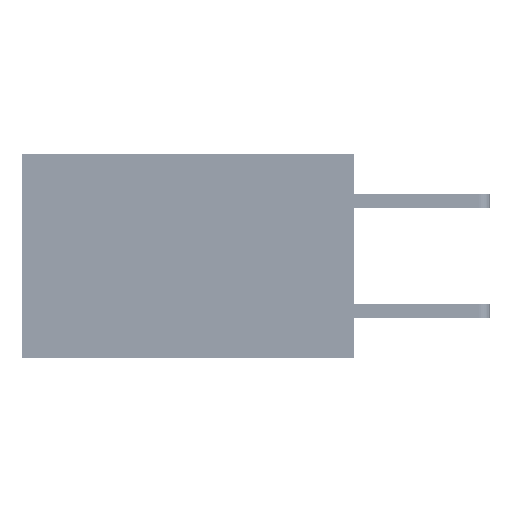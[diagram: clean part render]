
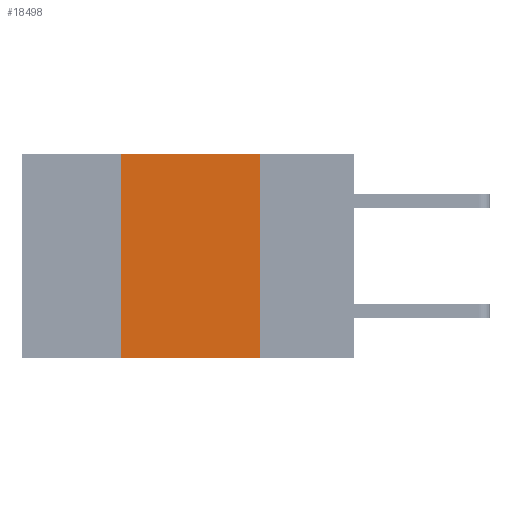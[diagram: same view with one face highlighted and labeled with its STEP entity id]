
A CAD part, left-side view. The second image highlights one B-rep face of the part: STEP entity #18498.
In plain terms, the highlighted planar face has unit normal (-1, 0, 0).
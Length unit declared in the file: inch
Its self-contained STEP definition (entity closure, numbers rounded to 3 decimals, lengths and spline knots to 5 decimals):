
#90 = LINE ( 'NONE', #34822, #17139 ) ;
#1323 = CARTESIAN_POINT ( 'NONE',  ( 0., 0.17, 0. ) ) ;
#3475 = DIRECTION ( 'NONE',  ( 1., 0., 0. ) ) ;
#3822 = EDGE_CURVE ( 'NONE', #50063, #41217, #90, .T. ) ;
#6707 = DIRECTION ( 'NONE',  ( 0., -1., 0. ) ) ;
#9091 = AXIS2_PLACEMENT_3D ( 'NONE', #14913, #3475, #50179 ) ;
#12660 = EDGE_CURVE ( 'NONE', #41217, #47361, #46963, .T. ) ;
#13399 = EDGE_CURVE ( 'NONE', #50063, #32348, #36809, .T. ) ;
#14913 = CARTESIAN_POINT ( 'NONE',  ( 0., 0.6, 0. ) ) ;
#15316 = DIRECTION ( 'NONE',  ( 0., -1., 0. ) ) ;
#17139 = VECTOR ( 'NONE', #49653, 39.37008 ) ;
#18024 = ORIENTED_EDGE ( 'NONE', *, *, #44090, .F. ) ;
#18498 = ADVANCED_FACE ( 'NONE', ( #37537 ), #22883, .F. ) ;
#22883 = PLANE ( 'NONE',  #9091 ) ;
#25505 = VECTOR ( 'NONE', #28757, 39.37008 ) ;
#26933 = CARTESIAN_POINT ( 'NONE',  ( 0., 0.42, -0.37 ) ) ;
#27983 = EDGE_LOOP ( 'NONE', ( #18024, #40698, #28709, #28834 ) ) ;
#28709 = ORIENTED_EDGE ( 'NONE', *, *, #3822, .F. ) ;
#28757 = DIRECTION ( 'NONE',  ( 0., 0., -1. ) ) ;
#28834 = ORIENTED_EDGE ( 'NONE', *, *, #13399, .T. ) ;
#29513 = CARTESIAN_POINT ( 'NONE',  ( 0., 0.17, -0.37 ) ) ;
#30999 = LINE ( 'NONE', #1323, #25505 ) ;
#31850 = VECTOR ( 'NONE', #6707, 39.37008 ) ;
#32348 = VERTEX_POINT ( 'NONE', #29513 ) ;
#34822 = CARTESIAN_POINT ( 'NONE',  ( 0., 0.42, 0. ) ) ;
#35366 = VECTOR ( 'NONE', #15316, 39.37008 ) ;
#36809 = LINE ( 'NONE', #41684, #31850 ) ;
#37537 = FACE_OUTER_BOUND ( 'NONE', #27983, .T. ) ;
#38132 = CARTESIAN_POINT ( 'NONE',  ( 0., 0.6, 0. ) ) ;
#40698 = ORIENTED_EDGE ( 'NONE', *, *, #12660, .F. ) ;
#41217 = VERTEX_POINT ( 'NONE', #43571 ) ;
#41684 = CARTESIAN_POINT ( 'NONE',  ( 0., 0.6, -0.37 ) ) ;
#43571 = CARTESIAN_POINT ( 'NONE',  ( 0., 0.42, 0. ) ) ;
#44090 = EDGE_CURVE ( 'NONE', #47361, #32348, #30999, .T. ) ;
#46963 = LINE ( 'NONE', #38132, #35366 ) ;
#47361 = VERTEX_POINT ( 'NONE', #49921 ) ;
#49653 = DIRECTION ( 'NONE',  ( 0., 0., 1. ) ) ;
#49921 = CARTESIAN_POINT ( 'NONE',  ( 0., 0.17, 0. ) ) ;
#50063 = VERTEX_POINT ( 'NONE', #26933 ) ;
#50179 = DIRECTION ( 'NONE',  ( 0., 0., -1. ) ) ;
